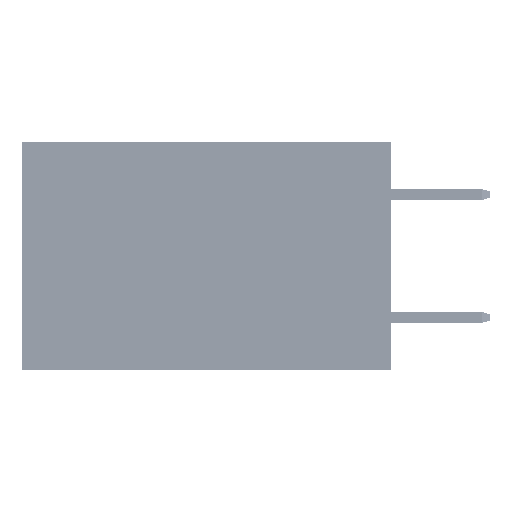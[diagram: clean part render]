
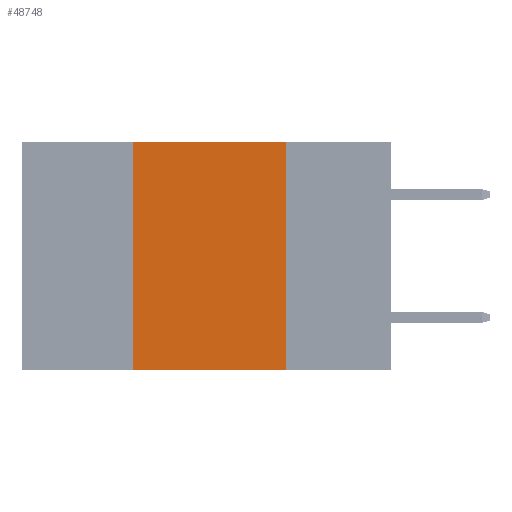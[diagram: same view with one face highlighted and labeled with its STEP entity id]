
A CAD part, left-side view. The second image highlights one B-rep face of the part: STEP entity #48748.
In plain terms, the highlighted planar face has unit normal (-1, 0, 0).
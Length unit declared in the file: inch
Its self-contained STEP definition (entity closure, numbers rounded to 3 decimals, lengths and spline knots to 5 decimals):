
#2571 = DIRECTION ( 'NONE',  ( 0., -1., 0. ) ) ;
#3027 = DIRECTION ( 'NONE',  ( 1., 0., 0. ) ) ;
#3794 = VERTEX_POINT ( 'NONE', #18298 ) ;
#6490 = CARTESIAN_POINT ( 'NONE',  ( 0., 0.42, 0. ) ) ;
#7160 = VERTEX_POINT ( 'NONE', #50085 ) ;
#7162 = EDGE_CURVE ( 'NONE', #11052, #3794, #48258, .T. ) ;
#8920 = CARTESIAN_POINT ( 'NONE',  ( 0., 0.6, -0.37 ) ) ;
#9927 = DIRECTION ( 'NONE',  ( 0., 0., -1. ) ) ;
#10243 = LINE ( 'NONE', #46628, #24520 ) ;
#11052 = VERTEX_POINT ( 'NONE', #6490 ) ;
#11453 = FACE_OUTER_BOUND ( 'NONE', #33868, .T. ) ;
#12925 = LINE ( 'NONE', #8920, #42771 ) ;
#14227 = VERTEX_POINT ( 'NONE', #46904 ) ;
#14244 = ORIENTED_EDGE ( 'NONE', *, *, #23825, .F. ) ;
#15722 = AXIS2_PLACEMENT_3D ( 'NONE', #24916, #3027, #46686 ) ;
#16556 = DIRECTION ( 'NONE',  ( 0., -1., 0. ) ) ;
#18298 = CARTESIAN_POINT ( 'NONE',  ( 0., 0.17, 0. ) ) ;
#19040 = DIRECTION ( 'NONE',  ( 0., 0., 1. ) ) ;
#19240 = VECTOR ( 'NONE', #9927, 39.37008 ) ;
#21067 = LINE ( 'NONE', #49322, #19240 ) ;
#21893 = EDGE_CURVE ( 'NONE', #14227, #7160, #12925, .T. ) ;
#23825 = EDGE_CURVE ( 'NONE', #3794, #7160, #21067, .T. ) ;
#24520 = VECTOR ( 'NONE', #19040, 39.37008 ) ;
#24916 = CARTESIAN_POINT ( 'NONE',  ( 0., 0.6, 0. ) ) ;
#26279 = CARTESIAN_POINT ( 'NONE',  ( 0., 0.6, 0. ) ) ;
#27789 = ORIENTED_EDGE ( 'NONE', *, *, #7162, .F. ) ;
#33868 = EDGE_LOOP ( 'NONE', ( #14244, #27789, #37021, #38893 ) ) ;
#34359 = EDGE_CURVE ( 'NONE', #14227, #11052, #10243, .T. ) ;
#37021 = ORIENTED_EDGE ( 'NONE', *, *, #34359, .F. ) ;
#37735 = VECTOR ( 'NONE', #2571, 39.37008 ) ;
#38893 = ORIENTED_EDGE ( 'NONE', *, *, #21893, .T. ) ;
#42771 = VECTOR ( 'NONE', #16556, 39.37008 ) ;
#46628 = CARTESIAN_POINT ( 'NONE',  ( 0., 0.42, 0. ) ) ;
#46686 = DIRECTION ( 'NONE',  ( 0., 0., -1. ) ) ;
#46904 = CARTESIAN_POINT ( 'NONE',  ( 0., 0.42, -0.37 ) ) ;
#48258 = LINE ( 'NONE', #26279, #37735 ) ;
#48672 = PLANE ( 'NONE',  #15722 ) ;
#48748 = ADVANCED_FACE ( 'NONE', ( #11453 ), #48672, .F. ) ;
#49322 = CARTESIAN_POINT ( 'NONE',  ( 0., 0.17, 0. ) ) ;
#50085 = CARTESIAN_POINT ( 'NONE',  ( 0., 0.17, -0.37 ) ) ;
